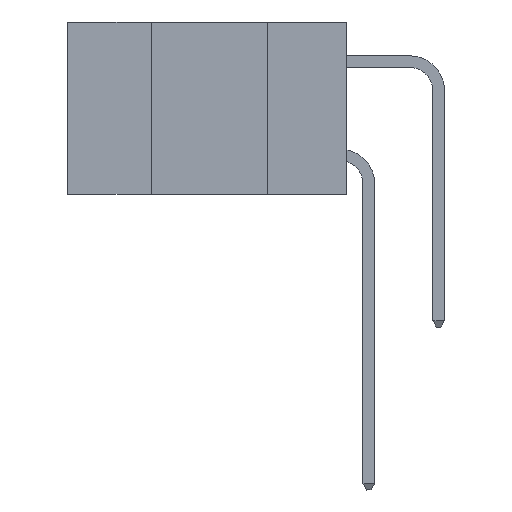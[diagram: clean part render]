
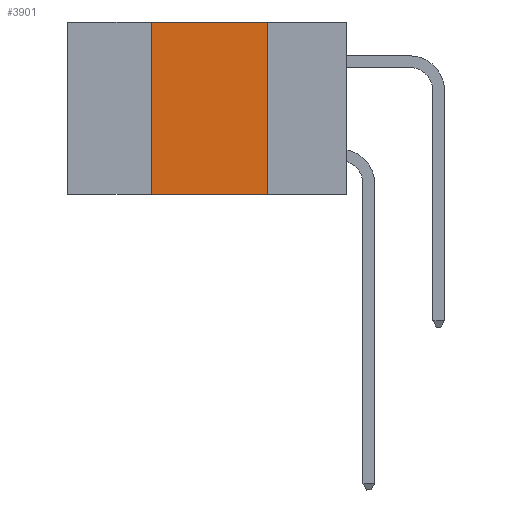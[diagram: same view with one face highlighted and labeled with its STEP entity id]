
A CAD part, left-side view. The second image highlights one B-rep face of the part: STEP entity #3901.
In plain terms, the highlighted planar face has unit normal (-1, 0, 0).
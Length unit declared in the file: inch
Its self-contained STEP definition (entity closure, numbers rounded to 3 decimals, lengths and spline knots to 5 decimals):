
#833 = CARTESIAN_POINT ( 'NONE',  ( 0., 0.17, 0. ) ) ;
#1240 = VERTEX_POINT ( 'NONE', #833 ) ;
#1306 = CARTESIAN_POINT ( 'NONE',  ( 0., 0.42, 0. ) ) ;
#1362 = CARTESIAN_POINT ( 'NONE',  ( 0., 0.42, 0. ) ) ;
#1809 = VERTEX_POINT ( 'NONE', #16972 ) ;
#3749 = EDGE_CURVE ( 'NONE', #1240, #6162, #11519, .T. ) ;
#3854 = VECTOR ( 'NONE', #12389, 39.37008 ) ;
#3901 = ADVANCED_FACE ( 'NONE', ( #5927 ), #12800, .F. ) ;
#4049 = ORIENTED_EDGE ( 'NONE', *, *, #4340, .F. ) ;
#4318 = VECTOR ( 'NONE', #7958, 39.37008 ) ;
#4333 = CARTESIAN_POINT ( 'NONE',  ( 0., 0.17, -0.37 ) ) ;
#4340 = EDGE_CURVE ( 'NONE', #1809, #17632, #7966, .T. ) ;
#4784 = LINE ( 'NONE', #5285, #3854 ) ;
#5137 = DIRECTION ( 'NONE',  ( 1., 0., 0. ) ) ;
#5285 = CARTESIAN_POINT ( 'NONE',  ( 0., 0.6, 0. ) ) ;
#5557 = DIRECTION ( 'NONE',  ( 0., 0., 1. ) ) ;
#5927 = FACE_OUTER_BOUND ( 'NONE', #16926, .T. ) ;
#6162 = VERTEX_POINT ( 'NONE', #4333 ) ;
#7958 = DIRECTION ( 'NONE',  ( 0., 0., -1. ) ) ;
#7966 = LINE ( 'NONE', #1306, #11485 ) ;
#8873 = CARTESIAN_POINT ( 'NONE',  ( 0., 0.6, -0.37 ) ) ;
#10084 = ORIENTED_EDGE ( 'NONE', *, *, #18487, .T. ) ;
#10792 = CARTESIAN_POINT ( 'NONE',  ( 0., 0.17, 0. ) ) ;
#11485 = VECTOR ( 'NONE', #5557, 39.37008 ) ;
#11519 = LINE ( 'NONE', #10792, #4318 ) ;
#11537 = AXIS2_PLACEMENT_3D ( 'NONE', #14026, #5137, #18508 ) ;
#12389 = DIRECTION ( 'NONE',  ( 0., -1., 0. ) ) ;
#12800 = PLANE ( 'NONE',  #11537 ) ;
#14026 = CARTESIAN_POINT ( 'NONE',  ( 0., 0.6, 0. ) ) ;
#14465 = ORIENTED_EDGE ( 'NONE', *, *, #3749, .F. ) ;
#16753 = EDGE_CURVE ( 'NONE', #17632, #1240, #4784, .T. ) ;
#16926 = EDGE_LOOP ( 'NONE', ( #14465, #18284, #4049, #10084 ) ) ;
#16972 = CARTESIAN_POINT ( 'NONE',  ( 0., 0.42, -0.37 ) ) ;
#17632 = VERTEX_POINT ( 'NONE', #1362 ) ;
#17692 = DIRECTION ( 'NONE',  ( 0., -1., 0. ) ) ;
#18284 = ORIENTED_EDGE ( 'NONE', *, *, #16753, .F. ) ;
#18334 = VECTOR ( 'NONE', #17692, 39.37008 ) ;
#18487 = EDGE_CURVE ( 'NONE', #1809, #6162, #19059, .T. ) ;
#18508 = DIRECTION ( 'NONE',  ( 0., 0., -1. ) ) ;
#19059 = LINE ( 'NONE', #8873, #18334 ) ;
